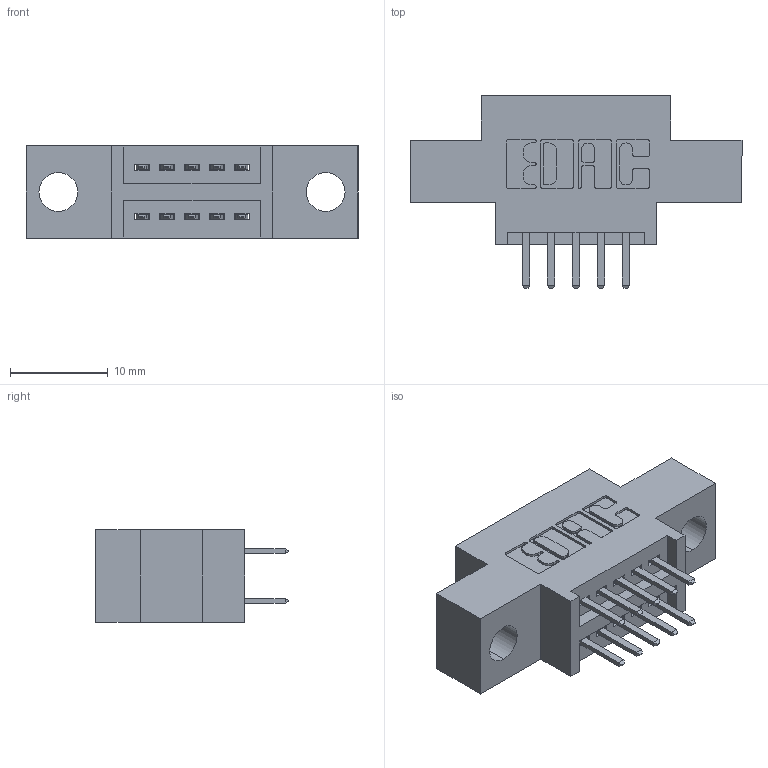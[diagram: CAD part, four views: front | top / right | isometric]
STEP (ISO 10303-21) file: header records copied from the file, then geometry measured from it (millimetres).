
FILE_DESCRIPTION (( 'STEP AP203' ), '1' );
FILE_NAME ('345-010-520-804.STEP', '2018-08-17T08:15:44', ( '' ), ( '' ), 'SwSTEP 2.0', 'SolidWorks 2016', '' );
FILE_SCHEMA (( 'CONFIG_CONTROL_DESIGN' ));
Length unit declared in the file: inch
Products named in the file (3): 345 Part_0.170 Offset - 0.156 Dia-TH; 345-292-001_345-293-120; 345-010-520-804
Assembly tree (11 placements, depth 2):
  345-010-520-804
    345 Part_0.170 Offset - 0.156 Dia-TH
    345-292-001_345-293-120  x10
Bounding box: 33.91 x 19.68 x 9.4 mm (x, y, z)
Volume: 2744.9 mm3; surface area: 3290.1 mm2
Topology: 11 solids, 11 shells, 670 faces, 1923 edges, 1254 vertices
Faces by surface type: plane 434, cylinder 236
Entity records: 9153 total; most frequent: CARTESIAN_POINT 1584, ORIENTED_EDGE 1506, DIRECTION 1429, EDGE_CURVE 753, LINE 597, VECTOR 597, VERTEX_POINT 498, AXIS2_PLACEMENT_3D 416
